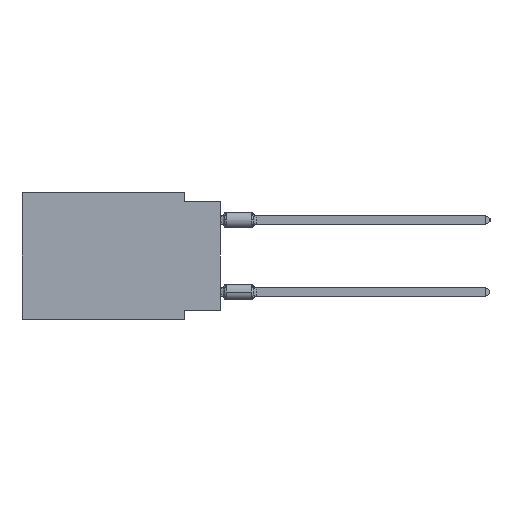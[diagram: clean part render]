
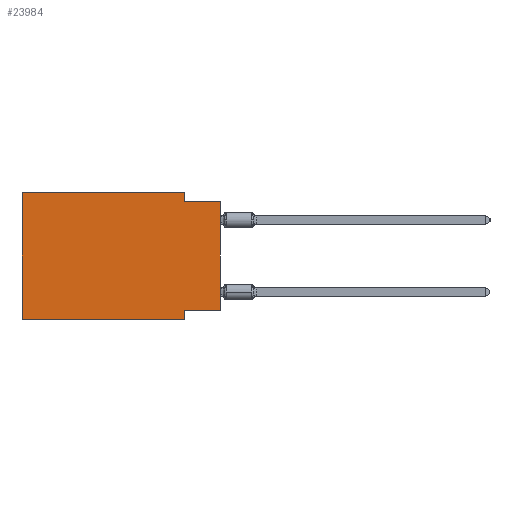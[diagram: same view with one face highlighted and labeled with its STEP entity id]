
A CAD part, left-side view. The second image highlights one B-rep face of the part: STEP entity #23984.
In plain terms, the highlighted planar face has unit normal (-1, 0, 0).
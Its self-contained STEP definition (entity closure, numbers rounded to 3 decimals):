
#409 = VERTEX_POINT ( 'NONE', #27054 ) ;
#907 = EDGE_CURVE ( 'NONE', #409, #32666, #36213, .T. ) ;
#1439 = EDGE_CURVE ( 'NONE', #6615, #34699, #15190, .T. ) ;
#1485 = EDGE_CURVE ( 'NONE', #409, #24481, #8264, .T. ) ;
#1516 = VECTOR ( 'NONE', #27585, 1000. ) ;
#1887 = CARTESIAN_POINT ( 'NONE',  ( 0., 13.97, -8.89 ) ) ;
#2207 = ORIENTED_EDGE ( 'NONE', *, *, #1485, .F. ) ;
#2814 = CARTESIAN_POINT ( 'NONE',  ( 0., 13.97, 0. ) ) ;
#2858 = PLANE ( 'NONE',  #13294 ) ;
#4123 = VERTEX_POINT ( 'NONE', #32458 ) ;
#5401 = DIRECTION ( 'NONE',  ( 0., 0., 1. ) ) ;
#6143 = VERTEX_POINT ( 'NONE', #9609 ) ;
#6205 = VECTOR ( 'NONE', #13775, 1000. ) ;
#6568 = ORIENTED_EDGE ( 'NONE', *, *, #24417, .F. ) ;
#6615 = VERTEX_POINT ( 'NONE', #27282 ) ;
#7376 = LINE ( 'NONE', #19439, #30179 ) ;
#7609 = CARTESIAN_POINT ( 'NONE',  ( 0., 2.54, 0. ) ) ;
#8264 = LINE ( 'NONE', #14814, #9884 ) ;
#9084 = DIRECTION ( 'NONE',  ( 1., 0., 0. ) ) ;
#9147 = CARTESIAN_POINT ( 'NONE',  ( 0., 0., -8.255 ) ) ;
#9609 = CARTESIAN_POINT ( 'NONE',  ( 0., 2.54, 0. ) ) ;
#9884 = VECTOR ( 'NONE', #21034, 1000. ) ;
#11248 = CARTESIAN_POINT ( 'NONE',  ( 0., 0., 0. ) ) ;
#11462 = ORIENTED_EDGE ( 'NONE', *, *, #33555, .F. ) ;
#11857 = LINE ( 'NONE', #29226, #21472 ) ;
#12227 = DIRECTION ( 'NONE',  ( 0., -1., 0. ) ) ;
#13294 = AXIS2_PLACEMENT_3D ( 'NONE', #14548, #9084, #23062 ) ;
#13775 = DIRECTION ( 'NONE',  ( 0., -1., 0. ) ) ;
#14548 = CARTESIAN_POINT ( 'NONE',  ( 0., 13.97, 0. ) ) ;
#14814 = CARTESIAN_POINT ( 'NONE',  ( 0., 13.97, 0. ) ) ;
#15093 = ORIENTED_EDGE ( 'NONE', *, *, #23397, .T. ) ;
#15190 = LINE ( 'NONE', #9147, #17090 ) ;
#15549 = CARTESIAN_POINT ( 'NONE',  ( 0., 2.54, -8.255 ) ) ;
#15861 = EDGE_LOOP ( 'NONE', ( #15093, #6568, #30501, #20201, #2207, #21679, #11462, #18214 ) ) ;
#17090 = VECTOR ( 'NONE', #20660, 1000. ) ;
#17344 = VECTOR ( 'NONE', #5401, 1000. ) ;
#18214 = ORIENTED_EDGE ( 'NONE', *, *, #1439, .F. ) ;
#18709 = DIRECTION ( 'NONE',  ( 0., -1., 0. ) ) ;
#19439 = CARTESIAN_POINT ( 'NONE',  ( 0., 0., -0.635 ) ) ;
#20201 = ORIENTED_EDGE ( 'NONE', *, *, #22100, .F. ) ;
#20660 = DIRECTION ( 'NONE',  ( 0., 1., 0. ) ) ;
#21034 = DIRECTION ( 'NONE',  ( 0., 0., 1. ) ) ;
#21428 = CARTESIAN_POINT ( 'NONE',  ( 0., 0., -0.635 ) ) ;
#21472 = VECTOR ( 'NONE', #12227, 1000. ) ;
#21679 = ORIENTED_EDGE ( 'NONE', *, *, #907, .T. ) ;
#22100 = EDGE_CURVE ( 'NONE', #24481, #6143, #11857, .T. ) ;
#23062 = DIRECTION ( 'NONE',  ( 0., 0., -1. ) ) ;
#23397 = EDGE_CURVE ( 'NONE', #6615, #32993, #31793, .T. ) ;
#23832 = EDGE_CURVE ( 'NONE', #6143, #4123, #25140, .T. ) ;
#23984 = ADVANCED_FACE ( 'NONE', ( #25512 ), #2858, .F. ) ;
#24417 = EDGE_CURVE ( 'NONE', #4123, #32993, #7376, .T. ) ;
#24481 = VERTEX_POINT ( 'NONE', #2814 ) ;
#24576 = LINE ( 'NONE', #33226, #1516 ) ;
#24835 = CARTESIAN_POINT ( 'NONE',  ( 0., 2.54, -8.89 ) ) ;
#25140 = LINE ( 'NONE', #7609, #31679 ) ;
#25512 = FACE_OUTER_BOUND ( 'NONE', #15861, .T. ) ;
#27054 = CARTESIAN_POINT ( 'NONE',  ( 0., 13.97, -8.89 ) ) ;
#27282 = CARTESIAN_POINT ( 'NONE',  ( 0., 0., -8.255 ) ) ;
#27585 = DIRECTION ( 'NONE',  ( 0., 0., -1. ) ) ;
#29226 = CARTESIAN_POINT ( 'NONE',  ( 0., 13.97, 0. ) ) ;
#30179 = VECTOR ( 'NONE', #18709, 1000. ) ;
#30501 = ORIENTED_EDGE ( 'NONE', *, *, #23832, .F. ) ;
#31679 = VECTOR ( 'NONE', #33620, 1000. ) ;
#31793 = LINE ( 'NONE', #11248, #17344 ) ;
#32458 = CARTESIAN_POINT ( 'NONE',  ( 0., 2.54, -0.635 ) ) ;
#32666 = VERTEX_POINT ( 'NONE', #24835 ) ;
#32993 = VERTEX_POINT ( 'NONE', #21428 ) ;
#33226 = CARTESIAN_POINT ( 'NONE',  ( 0., 2.54, -8.89 ) ) ;
#33555 = EDGE_CURVE ( 'NONE', #34699, #32666, #24576, .T. ) ;
#33620 = DIRECTION ( 'NONE',  ( 0., 0., -1. ) ) ;
#34699 = VERTEX_POINT ( 'NONE', #15549 ) ;
#36213 = LINE ( 'NONE', #1887, #6205 ) ;
